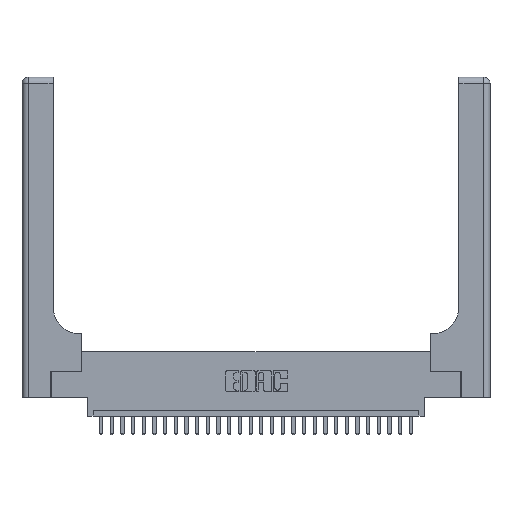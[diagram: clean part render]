
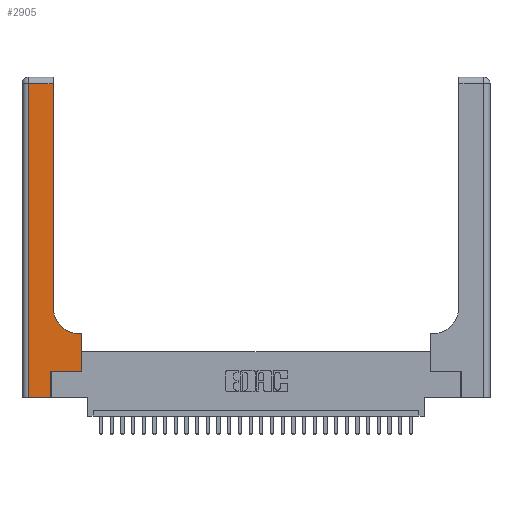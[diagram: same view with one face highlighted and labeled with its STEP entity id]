
A CAD part, top view. The second image highlights one B-rep face of the part: STEP entity #2905.
In plain terms, the highlighted planar face has unit normal (0, 0, 1).
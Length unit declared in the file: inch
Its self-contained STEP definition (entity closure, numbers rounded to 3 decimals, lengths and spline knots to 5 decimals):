
#535 = ORIENTED_EDGE ( 'NONE', *, *, #24521, .T. ) ;
#728 = ORIENTED_EDGE ( 'NONE', *, *, #22097, .T. ) ;
#1319 = CARTESIAN_POINT ( 'NONE',  ( 0.5415, 0.85, 0.37 ) ) ;
#1410 = EDGE_CURVE ( 'NONE', #6107, #10911, #18415, .T. ) ;
#1552 = FACE_OUTER_BOUND ( 'NONE', #26397, .T. ) ;
#1555 = LINE ( 'NONE', #7795, #27617 ) ;
#1984 = EDGE_CURVE ( 'NONE', #29005, #6107, #27357, .T. ) ;
#2096 = LINE ( 'NONE', #9940, #20281 ) ;
#2420 = VERTEX_POINT ( 'NONE', #15138 ) ;
#2905 = ADVANCED_FACE ( 'NONE', ( #1552 ), #23175, .F. ) ;
#3665 = CARTESIAN_POINT ( 'NONE',  ( 0.5585, 0.25, 0.37 ) ) ;
#3975 = VECTOR ( 'NONE', #12481, 39.37008 ) ;
#4454 = DIRECTION ( 'NONE',  ( 1., 0., 0. ) ) ;
#5099 = EDGE_CURVE ( 'NONE', #28733, #17775, #27882, .T. ) ;
#5206 = AXIS2_PLACEMENT_3D ( 'NONE', #1319, #12921, #8415 ) ;
#5420 = DIRECTION ( 'NONE',  ( 0., -1., 0. ) ) ;
#5668 = EDGE_CURVE ( 'NONE', #18215, #2420, #2096, .T. ) ;
#5951 = ORIENTED_EDGE ( 'NONE', *, *, #29092, .T. ) ;
#6107 = VERTEX_POINT ( 'NONE', #18602 ) ;
#6285 = DIRECTION ( 'NONE',  ( 0., 1., 0. ) ) ;
#7269 = DIRECTION ( 'NONE',  ( 0., 0., -1. ) ) ;
#7795 = CARTESIAN_POINT ( 'NONE',  ( 0.5585, 0.25, 0.37 ) ) ;
#7945 = ORIENTED_EDGE ( 'NONE', *, *, #1984, .T. ) ;
#7978 = LINE ( 'NONE', #16093, #27991 ) ;
#8415 = DIRECTION ( 'NONE',  ( 1., 0., 0. ) ) ;
#9672 = EDGE_CURVE ( 'NONE', #21736, #28733, #24366, .T. ) ;
#9940 = CARTESIAN_POINT ( 'NONE',  ( 0.06, 3., 0.37 ) ) ;
#10795 = CARTESIAN_POINT ( 'NONE',  ( 0.2915, 3., 0.37 ) ) ;
#10857 = DIRECTION ( 'NONE',  ( 0., 1., 0. ) ) ;
#10911 = VERTEX_POINT ( 'NONE', #3665 ) ;
#11203 = CARTESIAN_POINT ( 'NONE',  ( 0.06, 2.94, 0.37 ) ) ;
#11652 = CARTESIAN_POINT ( 'NONE',  ( 0.5585, 0.6, 0.37 ) ) ;
#12363 = LINE ( 'NONE', #10795, #14902 ) ;
#12481 = DIRECTION ( 'NONE',  ( -1., 0., 0. ) ) ;
#12921 = DIRECTION ( 'NONE',  ( 0., 0., -1. ) ) ;
#12974 = ORIENTED_EDGE ( 'NONE', *, *, #5668, .T. ) ;
#14301 = CARTESIAN_POINT ( 'NONE',  ( 0., 3., 0.37 ) ) ;
#14902 = VECTOR ( 'NONE', #24772, 39.37008 ) ;
#15138 = CARTESIAN_POINT ( 'NONE',  ( 0.06, 0., 0.37 ) ) ;
#15199 = ORIENTED_EDGE ( 'NONE', *, *, #9672, .T. ) ;
#15301 = EDGE_CURVE ( 'NONE', #17775, #21621, #12363, .T. ) ;
#16093 = CARTESIAN_POINT ( 'NONE',  ( 0., 0., 0.37 ) ) ;
#16653 = AXIS2_PLACEMENT_3D ( 'NONE', #14301, #7269, #19268 ) ;
#17293 = CARTESIAN_POINT ( 'NONE',  ( 0.269, 0., 0.37 ) ) ;
#17320 = VECTOR ( 'NONE', #10857, 39.37008 ) ;
#17716 = VECTOR ( 'NONE', #4454, 39.37008 ) ;
#17775 = VERTEX_POINT ( 'NONE', #18591 ) ;
#18041 = ORIENTED_EDGE ( 'NONE', *, *, #15301, .T. ) ;
#18215 = VERTEX_POINT ( 'NONE', #11203 ) ;
#18415 = LINE ( 'NONE', #27236, #17716 ) ;
#18591 = CARTESIAN_POINT ( 'NONE',  ( 0.2915, 0.85, 0.37 ) ) ;
#18602 = CARTESIAN_POINT ( 'NONE',  ( 0.269, 0.25, 0.37 ) ) ;
#19268 = DIRECTION ( 'NONE',  ( -1., 0., 0. ) ) ;
#20139 = CARTESIAN_POINT ( 'NONE',  ( 0.2915, 2.94, 0.37 ) ) ;
#20281 = VECTOR ( 'NONE', #5420, 39.37008 ) ;
#20754 = CARTESIAN_POINT ( 'NONE',  ( 0., 2.94, 0.37 ) ) ;
#20757 = ORIENTED_EDGE ( 'NONE', *, *, #5099, .T. ) ;
#20885 = CARTESIAN_POINT ( 'NONE',  ( 0.5415, 0.6, 0.37 ) ) ;
#21621 = VERTEX_POINT ( 'NONE', #20139 ) ;
#21700 = LINE ( 'NONE', #20754, #29607 ) ;
#21736 = VERTEX_POINT ( 'NONE', #11652 ) ;
#21780 = CARTESIAN_POINT ( 'NONE',  ( 0.269, 0., 0.37 ) ) ;
#21947 = CARTESIAN_POINT ( 'NONE',  ( 0.2915, 0.6, 0.37 ) ) ;
#22097 = EDGE_CURVE ( 'NONE', #21621, #18215, #21700, .T. ) ;
#23157 = DIRECTION ( 'NONE',  ( -1., 0., 0. ) ) ;
#23175 = PLANE ( 'NONE',  #16653 ) ;
#24366 = LINE ( 'NONE', #21947, #3975 ) ;
#24521 = EDGE_CURVE ( 'NONE', #2420, #29005, #7978, .T. ) ;
#24772 = DIRECTION ( 'NONE',  ( 0., 1., 0. ) ) ;
#26113 = ORIENTED_EDGE ( 'NONE', *, *, #1410, .T. ) ;
#26397 = EDGE_LOOP ( 'NONE', ( #18041, #728, #12974, #535, #7945, #26113, #5951, #15199, #20757 ) ) ;
#27236 = CARTESIAN_POINT ( 'NONE',  ( 0.269, 0.25, 0.37 ) ) ;
#27357 = LINE ( 'NONE', #17293, #17320 ) ;
#27488 = DIRECTION ( 'NONE',  ( 1., 0., 0. ) ) ;
#27617 = VECTOR ( 'NONE', #6285, 39.37008 ) ;
#27882 = CIRCLE ( 'NONE', #5206, 0.25 ) ;
#27991 = VECTOR ( 'NONE', #27488, 39.37008 ) ;
#28733 = VERTEX_POINT ( 'NONE', #20885 ) ;
#29005 = VERTEX_POINT ( 'NONE', #21780 ) ;
#29092 = EDGE_CURVE ( 'NONE', #10911, #21736, #1555, .T. ) ;
#29607 = VECTOR ( 'NONE', #23157, 39.37008 ) ;
